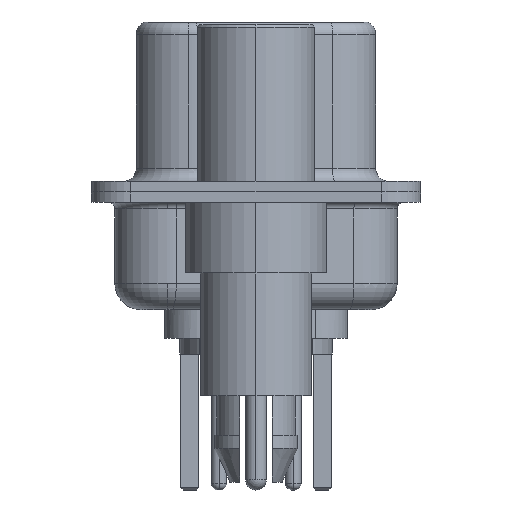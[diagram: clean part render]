
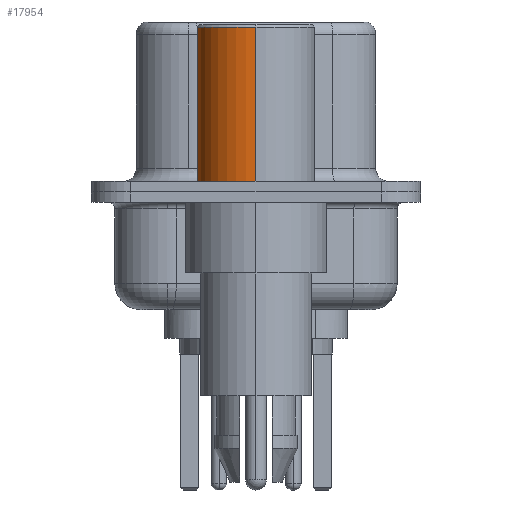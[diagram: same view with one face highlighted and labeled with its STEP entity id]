
A CAD part, left-side view. The second image highlights one B-rep face of the part: STEP entity #17954.
In plain terms, the highlighted cylindrical face has radius 2.25 mm (diameter 4.5 mm), a partial arc.
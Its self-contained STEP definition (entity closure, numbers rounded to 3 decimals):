
#830 = DIRECTION ( 'NONE',  ( 0., 0., 1. ) ) ;
#929 = EDGE_CURVE ( 'NONE', #20524, #20546, #15539, .T. ) ;
#1571 = VECTOR ( 'NONE', #11505, 1000. ) ;
#1771 = CIRCLE ( 'NONE', #18911, 2.25 ) ;
#4199 = ORIENTED_EDGE ( 'NONE', *, *, #4514, .T. ) ;
#4352 = DIRECTION ( 'NONE',  ( 0., 0., 1. ) ) ;
#4514 = EDGE_CURVE ( 'NONE', #10734, #7224, #12091, .T. ) ;
#4628 = FACE_OUTER_BOUND ( 'NONE', #17477, .T. ) ;
#7127 = CARTESIAN_POINT ( 'NONE',  ( 2.25, 0., 0.581 ) ) ;
#7224 = VERTEX_POINT ( 'NONE', #22516 ) ;
#7980 = DIRECTION ( 'NONE',  ( 0., 0., 1. ) ) ;
#8018 = AXIS2_PLACEMENT_3D ( 'NONE', #18857, #7980, #20568 ) ;
#8053 = CARTESIAN_POINT ( 'NONE',  ( 0., 0., 0.581 ) ) ;
#8515 = ORIENTED_EDGE ( 'NONE', *, *, #929, .F. ) ;
#9908 = DIRECTION ( 'NONE',  ( 1., 0., 0. ) ) ;
#10734 = VERTEX_POINT ( 'NONE', #20504 ) ;
#11505 = DIRECTION ( 'NONE',  ( 0., 0., 1. ) ) ;
#11674 = CARTESIAN_POINT ( 'NONE',  ( 0., 0., 0.4 ) ) ;
#11854 = EDGE_CURVE ( 'NONE', #20524, #10734, #1771, .T. ) ;
#12091 = LINE ( 'NONE', #17387, #20508 ) ;
#13545 = DIRECTION ( 'NONE',  ( 1., 0., 0. ) ) ;
#14906 = ORIENTED_EDGE ( 'NONE', *, *, #11854, .T. ) ;
#15539 = LINE ( 'NONE', #7127, #1571 ) ;
#15544 = EDGE_CURVE ( 'NONE', #20546, #7224, #21618, .T. ) ;
#17387 = CARTESIAN_POINT ( 'NONE',  ( -2.25, 0., 0.581 ) ) ;
#17477 = EDGE_LOOP ( 'NONE', ( #14906, #4199, #19987, #8515 ) ) ;
#17954 = ADVANCED_FACE ( 'NONE', ( #4628 ), #22619, .T. ) ;
#18135 = AXIS2_PLACEMENT_3D ( 'NONE', #8053, #4352, #9908 ) ;
#18857 = CARTESIAN_POINT ( 'NONE',  ( 0., 0., 6.3 ) ) ;
#18911 = AXIS2_PLACEMENT_3D ( 'NONE', #11674, #830, #13545 ) ;
#19114 = CARTESIAN_POINT ( 'NONE',  ( 2.25, 0., 0.4 ) ) ;
#19488 = CARTESIAN_POINT ( 'NONE',  ( 2.25, 0., 6.3 ) ) ;
#19851 = DIRECTION ( 'NONE',  ( 0., 0., 1. ) ) ;
#19987 = ORIENTED_EDGE ( 'NONE', *, *, #15544, .F. ) ;
#20504 = CARTESIAN_POINT ( 'NONE',  ( -2.25, 0., 0.4 ) ) ;
#20508 = VECTOR ( 'NONE', #19851, 1000. ) ;
#20524 = VERTEX_POINT ( 'NONE', #19114 ) ;
#20546 = VERTEX_POINT ( 'NONE', #19488 ) ;
#20568 = DIRECTION ( 'NONE',  ( 1., 0., 0. ) ) ;
#21618 = CIRCLE ( 'NONE', #8018, 2.25 ) ;
#22516 = CARTESIAN_POINT ( 'NONE',  ( -2.25, 0., 6.3 ) ) ;
#22619 = CYLINDRICAL_SURFACE ( 'NONE', #18135, 2.25 ) ;
